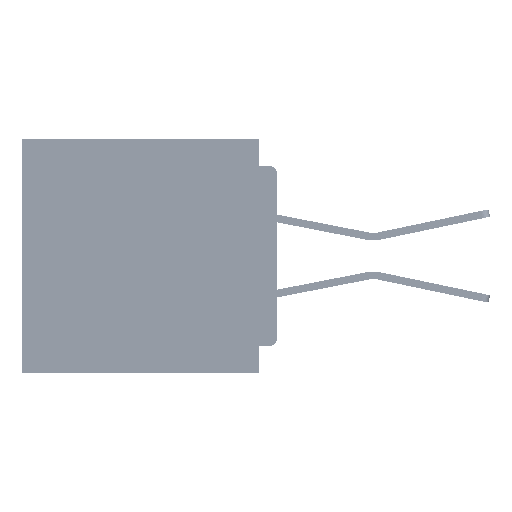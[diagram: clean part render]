
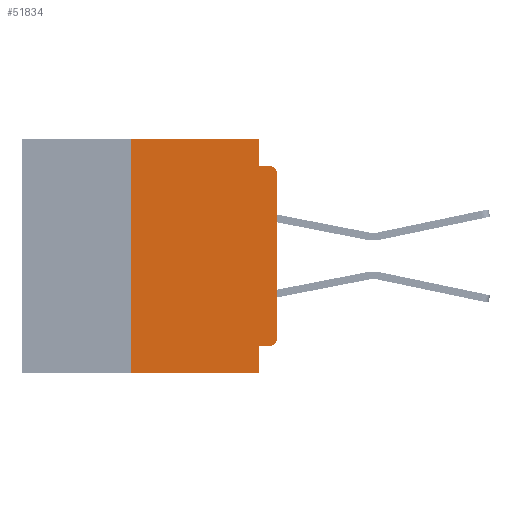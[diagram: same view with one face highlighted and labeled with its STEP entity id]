
A CAD part, left-side view. The second image highlights one B-rep face of the part: STEP entity #51834.
In plain terms, the highlighted planar face has unit normal (-1, 0, 0).
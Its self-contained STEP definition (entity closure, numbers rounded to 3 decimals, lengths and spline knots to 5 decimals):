
#338 = DIRECTION ( 'NONE',  ( 0., 0., -1. ) ) ;
#1687 = CARTESIAN_POINT ( 'NONE',  ( 0., 0.25, -0.4 ) ) ;
#2638 = VECTOR ( 'NONE', #39421, 39.37008 ) ;
#3721 = CARTESIAN_POINT ( 'NONE',  ( 0., 0.031, -0.4 ) ) ;
#3968 = CARTESIAN_POINT ( 'NONE',  ( 0., 0.015, -0.06 ) ) ;
#4183 = VECTOR ( 'NONE', #9149, 39.37008 ) ;
#4765 = CARTESIAN_POINT ( 'NONE',  ( 0., 0., -0.06 ) ) ;
#5886 = AXIS2_PLACEMENT_3D ( 'NONE', #42388, #10147, #47805 ) ;
#5910 = EDGE_CURVE ( 'NONE', #41404, #53763, #12576, .T. ) ;
#6432 = CARTESIAN_POINT ( 'NONE',  ( 0., 0., 0. ) ) ;
#7694 = CARTESIAN_POINT ( 'NONE',  ( 0., 0.031, -0.045 ) ) ;
#8234 = CARTESIAN_POINT ( 'NONE',  ( 0., 0.031, -0.355 ) ) ;
#9149 = DIRECTION ( 'NONE',  ( 0., 0., -1. ) ) ;
#9184 = EDGE_CURVE ( 'NONE', #21128, #56522, #68349, .T. ) ;
#9419 = DIRECTION ( 'NONE',  ( 0., 0., -1. ) ) ;
#9938 = EDGE_CURVE ( 'NONE', #14028, #22102, #49836, .T. ) ;
#10147 = DIRECTION ( 'NONE',  ( -1., 0., 0. ) ) ;
#10219 = PLANE ( 'NONE',  #12177 ) ;
#10428 = EDGE_CURVE ( 'NONE', #66927, #62599, #17796, .T. ) ;
#10674 = CARTESIAN_POINT ( 'NONE',  ( 0., 0., -0.355 ) ) ;
#11868 = DIRECTION ( 'NONE',  ( 0., 0., 1. ) ) ;
#12177 = AXIS2_PLACEMENT_3D ( 'NONE', #42454, #15655, #53262 ) ;
#12576 = LINE ( 'NONE', #10674, #39516 ) ;
#14028 = VERTEX_POINT ( 'NONE', #38300 ) ;
#15190 = CARTESIAN_POINT ( 'NONE',  ( 0., 0.437, -0.4 ) ) ;
#15365 = LINE ( 'NONE', #1687, #2638 ) ;
#15655 = DIRECTION ( 'NONE',  ( 1., 0., 0. ) ) ;
#16446 = CARTESIAN_POINT ( 'NONE',  ( 0., 0.031, 0. ) ) ;
#17079 = AXIS2_PLACEMENT_3D ( 'NONE', #3968, #41661, #9419 ) ;
#17796 = LINE ( 'NONE', #15190, #44703 ) ;
#20323 = EDGE_CURVE ( 'NONE', #41055, #14028, #38515, .T. ) ;
#21046 = ORIENTED_EDGE ( 'NONE', *, *, #45795, .T. ) ;
#21128 = VERTEX_POINT ( 'NONE', #4765 ) ;
#21441 = CARTESIAN_POINT ( 'NONE',  ( 0., 0.25, -0.4 ) ) ;
#22102 = VERTEX_POINT ( 'NONE', #7694 ) ;
#22777 = DIRECTION ( 'NONE',  ( 0., -1., 0. ) ) ;
#24087 = ORIENTED_EDGE ( 'NONE', *, *, #42094, .T. ) ;
#25931 = LINE ( 'NONE', #6432, #54523 ) ;
#25996 = DIRECTION ( 'NONE',  ( 0., -1., 0. ) ) ;
#26454 = DIRECTION ( 'NONE',  ( 0., 1., 0. ) ) ;
#28054 = CARTESIAN_POINT ( 'NONE',  ( 0., 0.031, -0.4 ) ) ;
#28171 = CARTESIAN_POINT ( 'NONE',  ( 0., 0.25, 0. ) ) ;
#29844 = DIRECTION ( 'NONE',  ( 0., -1., 0. ) ) ;
#31214 = ORIENTED_EDGE ( 'NONE', *, *, #55217, .F. ) ;
#33821 = VECTOR ( 'NONE', #338, 39.37008 ) ;
#35601 = CARTESIAN_POINT ( 'NONE',  ( 0., 0., -0.34 ) ) ;
#36680 = VERTEX_POINT ( 'NONE', #35601 ) ;
#37481 = EDGE_LOOP ( 'NONE', ( #21046, #63667, #41377, #59560, #46476, #44528, #42767, #31214, #50436, #24087 ) ) ;
#38145 = EDGE_CURVE ( 'NONE', #66927, #41055, #15365, .T. ) ;
#38300 = CARTESIAN_POINT ( 'NONE',  ( 0., 0.031, 0. ) ) ;
#38515 = LINE ( 'NONE', #56596, #67034 ) ;
#39421 = DIRECTION ( 'NONE',  ( 0., 0., 1. ) ) ;
#39516 = VECTOR ( 'NONE', #26454, 39.37008 ) ;
#41055 = VERTEX_POINT ( 'NONE', #28171 ) ;
#41377 = ORIENTED_EDGE ( 'NONE', *, *, #42886, .F. ) ;
#41404 = VERTEX_POINT ( 'NONE', #63114 ) ;
#41661 = DIRECTION ( 'NONE',  ( -1., 0., 0. ) ) ;
#42094 = EDGE_CURVE ( 'NONE', #41404, #36680, #69184, .T. ) ;
#42388 = CARTESIAN_POINT ( 'NONE',  ( 0., 0.015, -0.34 ) ) ;
#42454 = CARTESIAN_POINT ( 'NONE',  ( 0., 0.437, 0. ) ) ;
#42767 = ORIENTED_EDGE ( 'NONE', *, *, #10428, .T. ) ;
#42886 = EDGE_CURVE ( 'NONE', #22102, #56522, #48290, .T. ) ;
#44168 = CARTESIAN_POINT ( 'NONE',  ( 0., 0., -0.045 ) ) ;
#44528 = ORIENTED_EDGE ( 'NONE', *, *, #38145, .F. ) ;
#44703 = VECTOR ( 'NONE', #25996, 39.37008 ) ;
#45795 = EDGE_CURVE ( 'NONE', #36680, #21128, #25931, .T. ) ;
#46476 = ORIENTED_EDGE ( 'NONE', *, *, #20323, .F. ) ;
#47169 = LINE ( 'NONE', #3721, #4183 ) ;
#47805 = DIRECTION ( 'NONE',  ( 0., 0., -1. ) ) ;
#48290 = LINE ( 'NONE', #44168, #60840 ) ;
#49836 = LINE ( 'NONE', #16446, #33821 ) ;
#50436 = ORIENTED_EDGE ( 'NONE', *, *, #5910, .F. ) ;
#51834 = ADVANCED_FACE ( 'NONE', ( #53846 ), #10219, .F. ) ;
#53262 = DIRECTION ( 'NONE',  ( 0., 0., -1. ) ) ;
#53763 = VERTEX_POINT ( 'NONE', #8234 ) ;
#53846 = FACE_OUTER_BOUND ( 'NONE', #37481, .T. ) ;
#54523 = VECTOR ( 'NONE', #11868, 39.37008 ) ;
#55217 = EDGE_CURVE ( 'NONE', #53763, #62599, #47169, .T. ) ;
#56522 = VERTEX_POINT ( 'NONE', #63062 ) ;
#56596 = CARTESIAN_POINT ( 'NONE',  ( 0., 0.437, 0. ) ) ;
#59560 = ORIENTED_EDGE ( 'NONE', *, *, #9938, .F. ) ;
#60840 = VECTOR ( 'NONE', #22777, 39.37008 ) ;
#62599 = VERTEX_POINT ( 'NONE', #28054 ) ;
#63062 = CARTESIAN_POINT ( 'NONE',  ( 0., 0.015, -0.045 ) ) ;
#63114 = CARTESIAN_POINT ( 'NONE',  ( 0., 0.015, -0.355 ) ) ;
#63667 = ORIENTED_EDGE ( 'NONE', *, *, #9184, .T. ) ;
#66927 = VERTEX_POINT ( 'NONE', #21441 ) ;
#67034 = VECTOR ( 'NONE', #29844, 39.37008 ) ;
#68349 = CIRCLE ( 'NONE', #17079, 0.015 ) ;
#69184 = CIRCLE ( 'NONE', #5886, 0.015 ) ;
